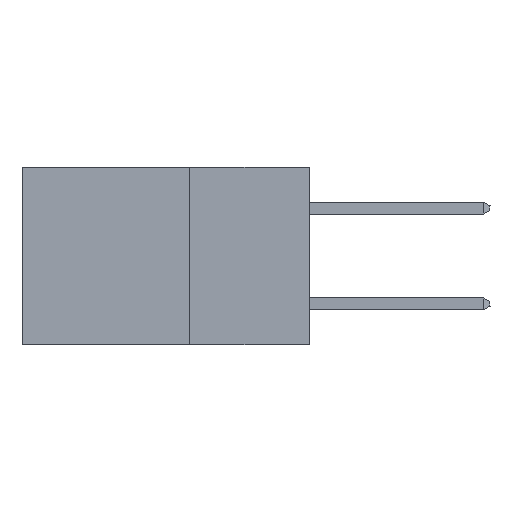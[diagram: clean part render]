
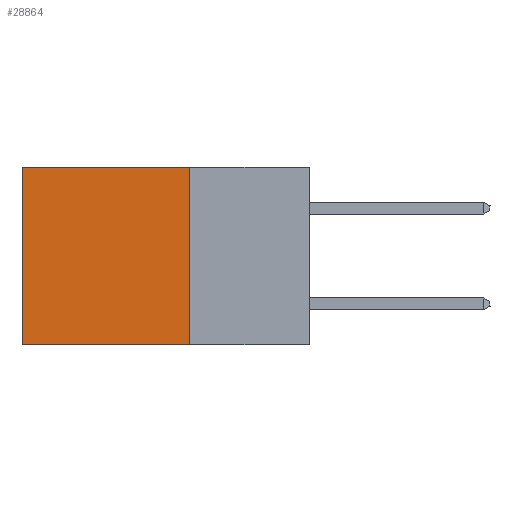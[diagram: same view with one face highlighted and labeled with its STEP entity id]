
A CAD part, left-side view. The second image highlights one B-rep face of the part: STEP entity #28864.
In plain terms, the highlighted planar face has unit normal (-1, 0, 0).
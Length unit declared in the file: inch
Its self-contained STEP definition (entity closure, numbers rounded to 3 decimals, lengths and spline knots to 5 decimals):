
#788 = CARTESIAN_POINT ( 'NONE',  ( 0.2875, 0.25, 0. ) ) ;
#998 = EDGE_CURVE ( 'NONE', #21593, #2900, #27802, .T. ) ;
#1349 = ORIENTED_EDGE ( 'NONE', *, *, #998, .F. ) ;
#1408 = CARTESIAN_POINT ( 'NONE',  ( 0.2875, 0.6, 0. ) ) ;
#2802 = ORIENTED_EDGE ( 'NONE', *, *, #28910, .T. ) ;
#2900 = VERTEX_POINT ( 'NONE', #40055 ) ;
#3979 = DIRECTION ( 'NONE',  ( 0., 0., -1. ) ) ;
#5322 = CARTESIAN_POINT ( 'NONE',  ( 0.2875, 0.25, -0.37 ) ) ;
#5619 = VECTOR ( 'NONE', #32268, 39.37008 ) ;
#6680 = VECTOR ( 'NONE', #39188, 39.37008 ) ;
#9454 = VERTEX_POINT ( 'NONE', #26031 ) ;
#11154 = LINE ( 'NONE', #35561, #6680 ) ;
#11515 = CARTESIAN_POINT ( 'NONE',  ( 0.2875, 0.25, 0. ) ) ;
#12097 = DIRECTION ( 'NONE',  ( 0., 1., 0. ) ) ;
#12869 = CARTESIAN_POINT ( 'NONE',  ( 0.2875, 0.25, 0. ) ) ;
#13518 = LINE ( 'NONE', #1408, #5619 ) ;
#13689 = DIRECTION ( 'NONE',  ( 1., 0., 0. ) ) ;
#15783 = EDGE_LOOP ( 'NONE', ( #19826, #1349, #23304, #2802 ) ) ;
#18609 = AXIS2_PLACEMENT_3D ( 'NONE', #788, #13689, #3979 ) ;
#18971 = LINE ( 'NONE', #12869, #25824 ) ;
#19826 = ORIENTED_EDGE ( 'NONE', *, *, #40607, .T. ) ;
#21593 = VERTEX_POINT ( 'NONE', #5322 ) ;
#21770 = CARTESIAN_POINT ( 'NONE',  ( 0.2875, 0.25, -0.37 ) ) ;
#23304 = ORIENTED_EDGE ( 'NONE', *, *, #34284, .F. ) ;
#25287 = VECTOR ( 'NONE', #12097, 39.37008 ) ;
#25824 = VECTOR ( 'NONE', #40581, 39.37008 ) ;
#25886 = FACE_OUTER_BOUND ( 'NONE', #15783, .T. ) ;
#26031 = CARTESIAN_POINT ( 'NONE',  ( 0.2875, 0.6, 0. ) ) ;
#27802 = LINE ( 'NONE', #21770, #25287 ) ;
#28864 = ADVANCED_FACE ( 'NONE', ( #25886 ), #38608, .F. ) ;
#28910 = EDGE_CURVE ( 'NONE', #37345, #9454, #11154, .T. ) ;
#32268 = DIRECTION ( 'NONE',  ( 0., 0., -1. ) ) ;
#34284 = EDGE_CURVE ( 'NONE', #37345, #21593, #18971, .T. ) ;
#35561 = CARTESIAN_POINT ( 'NONE',  ( 0.2875, 0.25, 0. ) ) ;
#37345 = VERTEX_POINT ( 'NONE', #11515 ) ;
#38608 = PLANE ( 'NONE',  #18609 ) ;
#39188 = DIRECTION ( 'NONE',  ( 0., 1., 0. ) ) ;
#40055 = CARTESIAN_POINT ( 'NONE',  ( 0.2875, 0.6, -0.37 ) ) ;
#40581 = DIRECTION ( 'NONE',  ( 0., 0., -1. ) ) ;
#40607 = EDGE_CURVE ( 'NONE', #9454, #2900, #13518, .T. ) ;
